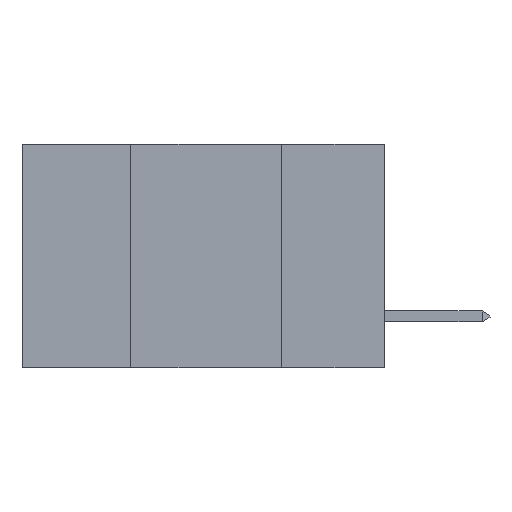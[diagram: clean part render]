
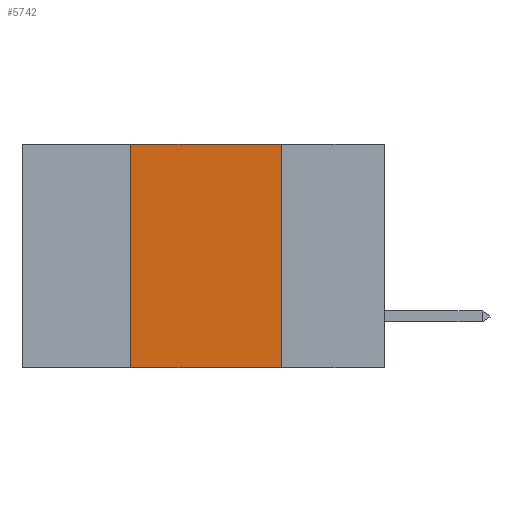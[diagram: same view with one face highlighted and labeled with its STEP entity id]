
A CAD part, left-side view. The second image highlights one B-rep face of the part: STEP entity #5742.
In plain terms, the highlighted planar face has unit normal (-1, 0, 0).
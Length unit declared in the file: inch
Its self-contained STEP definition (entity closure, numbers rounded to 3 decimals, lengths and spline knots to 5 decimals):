
#1647 = VECTOR ( 'NONE', #17766, 39.37008 ) ;
#2161 = VECTOR ( 'NONE', #11575, 39.37008 ) ;
#2898 = AXIS2_PLACEMENT_3D ( 'NONE', #3928, #7052, #28656 ) ;
#3928 = CARTESIAN_POINT ( 'NONE',  ( 0., 0.6, 0. ) ) ;
#4000 = EDGE_CURVE ( 'NONE', #35019, #32100, #11416, .T. ) ;
#4242 = EDGE_CURVE ( 'NONE', #8065, #32100, #10894, .T. ) ;
#5508 = CARTESIAN_POINT ( 'NONE',  ( 0., 0.17, -0.37 ) ) ;
#5742 = ADVANCED_FACE ( 'NONE', ( #20003 ), #22503, .F. ) ;
#7052 = DIRECTION ( 'NONE',  ( 1., 0., 0. ) ) ;
#8065 = VERTEX_POINT ( 'NONE', #27699 ) ;
#8881 = ORIENTED_EDGE ( 'NONE', *, *, #22943, .F. ) ;
#9940 = EDGE_LOOP ( 'NONE', ( #29014, #8881, #12742, #18544 ) ) ;
#10424 = VECTOR ( 'NONE', #16556, 39.37008 ) ;
#10894 = LINE ( 'NONE', #33039, #2161 ) ;
#11416 = LINE ( 'NONE', #25856, #10424 ) ;
#11575 = DIRECTION ( 'NONE',  ( 0., 0., -1. ) ) ;
#12742 = ORIENTED_EDGE ( 'NONE', *, *, #15226, .F. ) ;
#14429 = VERTEX_POINT ( 'NONE', #24675 ) ;
#14446 = DIRECTION ( 'NONE',  ( 0., 0., 1. ) ) ;
#15226 = EDGE_CURVE ( 'NONE', #35019, #14429, #38148, .T. ) ;
#16556 = DIRECTION ( 'NONE',  ( 0., -1., 0. ) ) ;
#17766 = DIRECTION ( 'NONE',  ( 0., -1., 0. ) ) ;
#18544 = ORIENTED_EDGE ( 'NONE', *, *, #4000, .T. ) ;
#19113 = LINE ( 'NONE', #39008, #1647 ) ;
#20003 = FACE_OUTER_BOUND ( 'NONE', #9940, .T. ) ;
#22503 = PLANE ( 'NONE',  #2898 ) ;
#22943 = EDGE_CURVE ( 'NONE', #14429, #8065, #19113, .T. ) ;
#24675 = CARTESIAN_POINT ( 'NONE',  ( 0., 0.42, 0. ) ) ;
#25856 = CARTESIAN_POINT ( 'NONE',  ( 0., 0.6, -0.37 ) ) ;
#27699 = CARTESIAN_POINT ( 'NONE',  ( 0., 0.17, 0. ) ) ;
#28656 = DIRECTION ( 'NONE',  ( 0., 0., -1. ) ) ;
#29014 = ORIENTED_EDGE ( 'NONE', *, *, #4242, .F. ) ;
#32100 = VERTEX_POINT ( 'NONE', #5508 ) ;
#33039 = CARTESIAN_POINT ( 'NONE',  ( 0., 0.17, 0. ) ) ;
#35019 = VERTEX_POINT ( 'NONE', #35027 ) ;
#35027 = CARTESIAN_POINT ( 'NONE',  ( 0., 0.42, -0.37 ) ) ;
#37202 = VECTOR ( 'NONE', #14446, 39.37008 ) ;
#38148 = LINE ( 'NONE', #38909, #37202 ) ;
#38909 = CARTESIAN_POINT ( 'NONE',  ( 0., 0.42, 0. ) ) ;
#39008 = CARTESIAN_POINT ( 'NONE',  ( 0., 0.6, 0. ) ) ;
